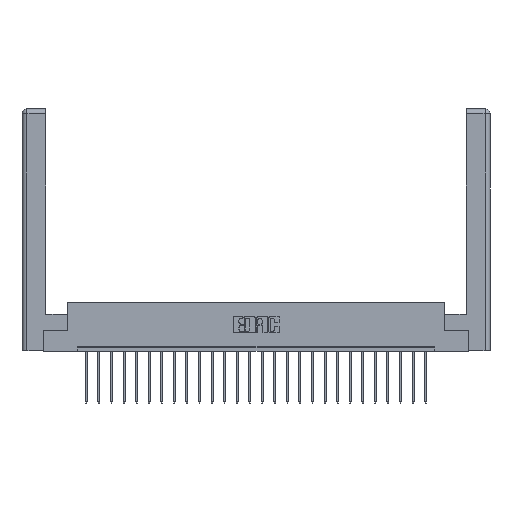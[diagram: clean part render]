
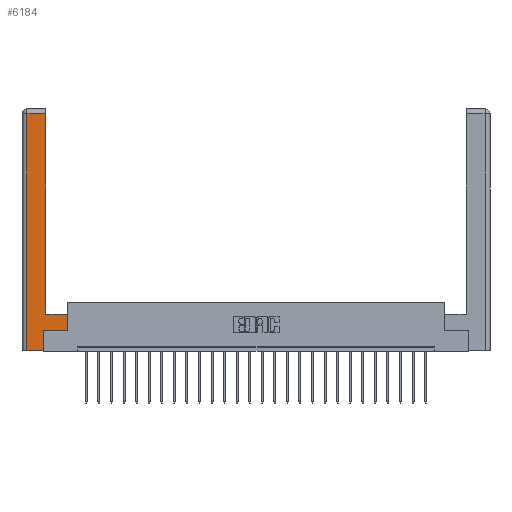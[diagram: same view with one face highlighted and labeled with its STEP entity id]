
A CAD part, top view. The second image highlights one B-rep face of the part: STEP entity #6184.
In plain terms, the highlighted planar face has unit normal (0, 0, 1).
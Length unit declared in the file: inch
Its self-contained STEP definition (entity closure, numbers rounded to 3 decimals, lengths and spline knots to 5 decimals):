
#50 = EDGE_CURVE ( 'NONE', #21903, #16188, #23959, .T. ) ;
#193 = LINE ( 'NONE', #8205, #19741 ) ;
#846 = ORIENTED_EDGE ( 'NONE', *, *, #12373, .T. ) ;
#847 = CARTESIAN_POINT ( 'NONE',  ( 0.295, 0.45, 0. ) ) ;
#991 = CARTESIAN_POINT ( 'NONE',  ( 0., 0., 0. ) ) ;
#1022 = CARTESIAN_POINT ( 'NONE',  ( 0.265, 0., 0. ) ) ;
#1344 = VECTOR ( 'NONE', #16758, 39.37008 ) ;
#1511 = CARTESIAN_POINT ( 'NONE',  ( 0.565, 0.45, 0. ) ) ;
#1672 = ORIENTED_EDGE ( 'NONE', *, *, #9745, .T. ) ;
#1913 = CARTESIAN_POINT ( 'NONE',  ( 0.295, 0.45, 0. ) ) ;
#1957 = CARTESIAN_POINT ( 'NONE',  ( 0.0615, 0., 0. ) ) ;
#2697 = CARTESIAN_POINT ( 'NONE',  ( 0.265, 0., 0. ) ) ;
#3268 = LINE ( 'NONE', #1913, #23418 ) ;
#3947 = DIRECTION ( 'NONE',  ( 0., 1., 0. ) ) ;
#4232 = ORIENTED_EDGE ( 'NONE', *, *, #7350, .T. ) ;
#5156 = EDGE_CURVE ( 'NONE', #14623, #21670, #17607, .T. ) ;
#6059 = CARTESIAN_POINT ( 'NONE',  ( 0.565, 0.45, 0. ) ) ;
#6080 = DIRECTION ( 'NONE',  ( -1., 0., 0. ) ) ;
#6184 = ADVANCED_FACE ( 'NONE', ( #10792 ), #16668, .F. ) ;
#6305 = VECTOR ( 'NONE', #8672, 39.37008 ) ;
#6307 = EDGE_CURVE ( 'NONE', #18275, #14623, #16598, .T. ) ;
#7065 = VECTOR ( 'NONE', #23371, 39.37008 ) ;
#7350 = EDGE_CURVE ( 'NONE', #18645, #21903, #19625, .T. ) ;
#8197 = VECTOR ( 'NONE', #9153, 39.37008 ) ;
#8205 = CARTESIAN_POINT ( 'NONE',  ( 0.265, 0.245, 0. ) ) ;
#8525 = ORIENTED_EDGE ( 'NONE', *, *, #24918, .T. ) ;
#8672 = DIRECTION ( 'NONE',  ( 1., 0., 0. ) ) ;
#8849 = ORIENTED_EDGE ( 'NONE', *, *, #50, .T. ) ;
#8880 = AXIS2_PLACEMENT_3D ( 'NONE', #991, #22418, #20613 ) ;
#9153 = DIRECTION ( 'NONE',  ( 0., 1., 0. ) ) ;
#9745 = EDGE_CURVE ( 'NONE', #23912, #22094, #25297, .T. ) ;
#10091 = VECTOR ( 'NONE', #20433, 39.37008 ) ;
#10157 = DIRECTION ( 'NONE',  ( 0., 1., 0. ) ) ;
#10792 = FACE_OUTER_BOUND ( 'NONE', #22114, .T. ) ;
#11367 = CARTESIAN_POINT ( 'NONE',  ( 0.565, 0.245, 0. ) ) ;
#12140 = CARTESIAN_POINT ( 'NONE',  ( 0.0615, 2.94, 0. ) ) ;
#12373 = EDGE_CURVE ( 'NONE', #21670, #18645, #193, .T. ) ;
#13883 = VECTOR ( 'NONE', #3947, 39.37008 ) ;
#14623 = VERTEX_POINT ( 'NONE', #1957 ) ;
#15293 = EDGE_CURVE ( 'NONE', #22094, #18275, #17753, .T. ) ;
#16188 = VERTEX_POINT ( 'NONE', #1511 ) ;
#16598 = LINE ( 'NONE', #20862, #1344 ) ;
#16668 = PLANE ( 'NONE',  #8880 ) ;
#16758 = DIRECTION ( 'NONE',  ( 0., -1., 0. ) ) ;
#17516 = CARTESIAN_POINT ( 'NONE',  ( 0.295, 2.94, 0. ) ) ;
#17607 = LINE ( 'NONE', #1022, #6305 ) ;
#17753 = LINE ( 'NONE', #18543, #10091 ) ;
#18275 = VERTEX_POINT ( 'NONE', #12140 ) ;
#18543 = CARTESIAN_POINT ( 'NONE',  ( 0.0615, 2.94, 0. ) ) ;
#18645 = VERTEX_POINT ( 'NONE', #20604 ) ;
#19008 = CARTESIAN_POINT ( 'NONE',  ( 0.295, 3., 0. ) ) ;
#19625 = LINE ( 'NONE', #21227, #7065 ) ;
#19741 = VECTOR ( 'NONE', #10157, 39.37008 ) ;
#20433 = DIRECTION ( 'NONE',  ( -1., 0., 0. ) ) ;
#20604 = CARTESIAN_POINT ( 'NONE',  ( 0.265, 0.245, 0. ) ) ;
#20613 = DIRECTION ( 'NONE',  ( -1., 0., 0. ) ) ;
#20736 = ORIENTED_EDGE ( 'NONE', *, *, #6307, .T. ) ;
#20862 = CARTESIAN_POINT ( 'NONE',  ( 0.0615, 0., 0. ) ) ;
#21227 = CARTESIAN_POINT ( 'NONE',  ( 0.565, 0.245, 0. ) ) ;
#21670 = VERTEX_POINT ( 'NONE', #2697 ) ;
#21903 = VERTEX_POINT ( 'NONE', #11367 ) ;
#22094 = VERTEX_POINT ( 'NONE', #17516 ) ;
#22114 = EDGE_LOOP ( 'NONE', ( #1672, #25179, #20736, #22527, #846, #4232, #8849, #8525 ) ) ;
#22418 = DIRECTION ( 'NONE',  ( 0., 0., -1. ) ) ;
#22527 = ORIENTED_EDGE ( 'NONE', *, *, #5156, .T. ) ;
#23371 = DIRECTION ( 'NONE',  ( 1., 0., 0. ) ) ;
#23418 = VECTOR ( 'NONE', #6080, 39.37008 ) ;
#23912 = VERTEX_POINT ( 'NONE', #847 ) ;
#23959 = LINE ( 'NONE', #6059, #13883 ) ;
#24918 = EDGE_CURVE ( 'NONE', #16188, #23912, #3268, .T. ) ;
#25179 = ORIENTED_EDGE ( 'NONE', *, *, #15293, .T. ) ;
#25297 = LINE ( 'NONE', #19008, #8197 ) ;
